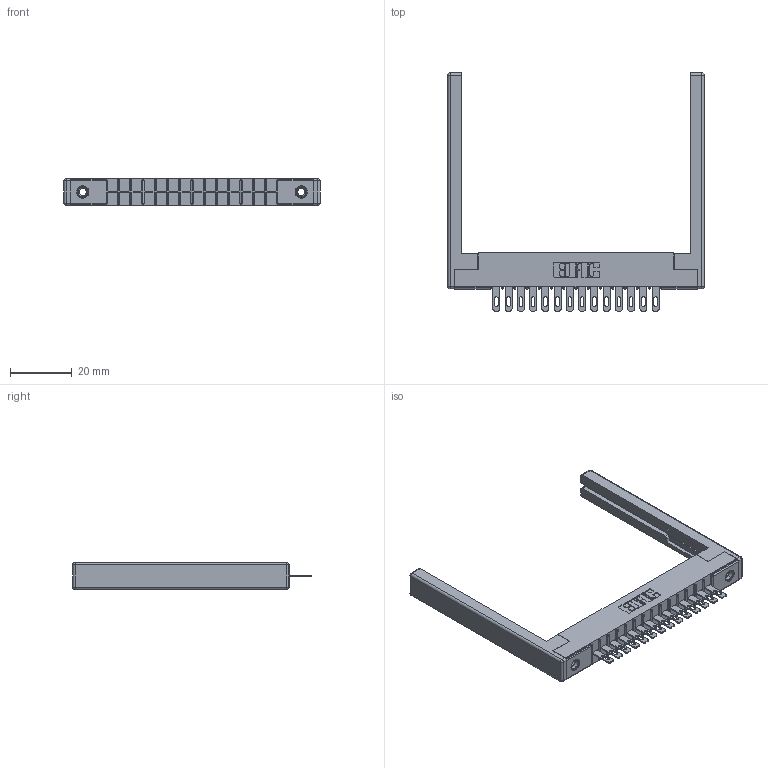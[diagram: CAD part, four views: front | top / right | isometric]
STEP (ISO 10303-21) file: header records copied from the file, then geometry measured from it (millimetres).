
FILE_DESCRIPTION (( 'STEP AP203' ), '1' );
FILE_NAME ('316-014-400-168.STEP', '2020-09-22T16:51:12', ( '' ), ( '' ), 'SwSTEP 2.0', 'SolidWorks 2020', '' );
FILE_SCHEMA (( 'CONFIG_CONTROL_DESIGN' ));
Length unit declared in the file: inch
Products named in the file (5): 316-014-400-168; 306-290-001_100; 307-220-068; 345-250-001_345-250-001-102; 306 Part_.156 Dia
Assembly tree (19 placements, depth 2):
  316-014-400-168
    306 Part_.156 Dia
    306-290-001_100  x14
    345-250-001_345-250-001-102  x2
    307-220-068  x2
Bounding box: 82.91 x 77.17 x 8.71 mm (x, y, z)
Volume: 10232.1 mm3; surface area: 12477.5 mm2
Topology: 19 solids, 19 shells, 1334 faces, 3716 edges, 2380 vertices
Faces by surface type: plane 856, cylinder 398, sphere 64, cone 12, torus 4
Entity records: 19606 total; most frequent: CARTESIAN_POINT 3254, DIRECTION 3225, ORIENTED_EDGE 3214, EDGE_CURVE 1607, VECTOR 1235, LINE 1235, VERTEX_POINT 1024, AXIS2_PLACEMENT_3D 995
